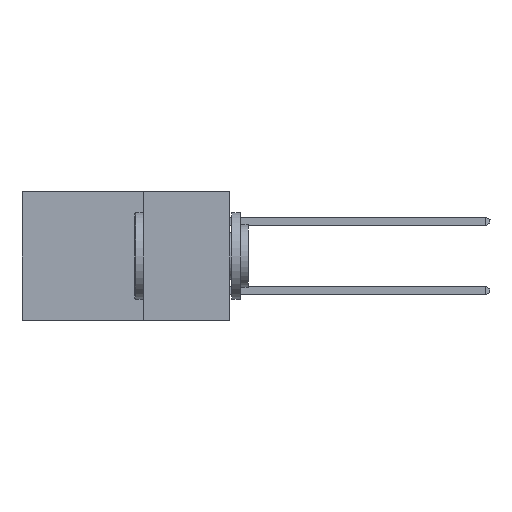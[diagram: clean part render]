
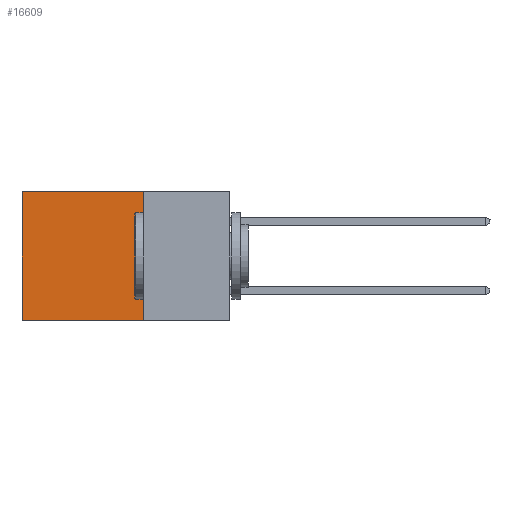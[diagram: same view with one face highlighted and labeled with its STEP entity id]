
A CAD part, left-side view. The second image highlights one B-rep face of the part: STEP entity #16609.
In plain terms, the highlighted planar face has unit normal (-1, 0, 0).
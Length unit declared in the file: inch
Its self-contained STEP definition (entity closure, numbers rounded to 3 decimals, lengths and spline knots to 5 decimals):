
#546 = DIRECTION ( 'NONE',  ( 0., 1., 0. ) ) ;
#1511 = EDGE_CURVE ( 'NONE', #17264, #19037, #10240, .T. ) ;
#3808 = CARTESIAN_POINT ( 'NONE',  ( 0.2615, 0.25, -0.37 ) ) ;
#4398 = VECTOR ( 'NONE', #15014, 39.37008 ) ;
#5291 = ORIENTED_EDGE ( 'NONE', *, *, #14490, .T. ) ;
#6304 = ORIENTED_EDGE ( 'NONE', *, *, #17550, .F. ) ;
#6436 = CARTESIAN_POINT ( 'NONE',  ( 0.2615, 0.6, -0.37 ) ) ;
#7663 = CARTESIAN_POINT ( 'NONE',  ( 0.2615, 0.25, -0.37 ) ) ;
#7667 = CARTESIAN_POINT ( 'NONE',  ( 0.2615, 0.25, 0. ) ) ;
#8010 = CARTESIAN_POINT ( 'NONE',  ( 0.2615, 0.6, 0. ) ) ;
#8348 = CARTESIAN_POINT ( 'NONE',  ( 0.2615, 0.25, 0. ) ) ;
#8584 = LINE ( 'NONE', #6436, #4398 ) ;
#10240 = LINE ( 'NONE', #3808, #11308 ) ;
#11308 = VECTOR ( 'NONE', #18964, 39.37008 ) ;
#12254 = CARTESIAN_POINT ( 'NONE',  ( 0.2615, 0.25, -0.37 ) ) ;
#12441 = VECTOR ( 'NONE', #546, 39.37008 ) ;
#12472 = LINE ( 'NONE', #27522, #13146 ) ;
#13146 = VECTOR ( 'NONE', #25366, 39.37008 ) ;
#13531 = AXIS2_PLACEMENT_3D ( 'NONE', #12254, #25421, #18827 ) ;
#14490 = EDGE_CURVE ( 'NONE', #25610, #26361, #8584, .T. ) ;
#15014 = DIRECTION ( 'NONE',  ( 0., 0., -1. ) ) ;
#15855 = CARTESIAN_POINT ( 'NONE',  ( 0.2615, 0.6, -0.37 ) ) ;
#16609 = ADVANCED_FACE ( 'NONE', ( #18974 ), #25133, .F. ) ;
#17264 = VERTEX_POINT ( 'NONE', #8348 ) ;
#17550 = EDGE_CURVE ( 'NONE', #19037, #26361, #12472, .T. ) ;
#18542 = LINE ( 'NONE', #7667, #12441 ) ;
#18827 = DIRECTION ( 'NONE',  ( 0., 0., -1. ) ) ;
#18964 = DIRECTION ( 'NONE',  ( 0., 0., -1. ) ) ;
#18974 = FACE_OUTER_BOUND ( 'NONE', #20964, .T. ) ;
#19037 = VERTEX_POINT ( 'NONE', #7663 ) ;
#20250 = EDGE_CURVE ( 'NONE', #17264, #25610, #18542, .T. ) ;
#20964 = EDGE_LOOP ( 'NONE', ( #5291, #6304, #23328, #22970 ) ) ;
#22970 = ORIENTED_EDGE ( 'NONE', *, *, #20250, .T. ) ;
#23328 = ORIENTED_EDGE ( 'NONE', *, *, #1511, .F. ) ;
#25133 = PLANE ( 'NONE',  #13531 ) ;
#25366 = DIRECTION ( 'NONE',  ( 0., 1., 0. ) ) ;
#25421 = DIRECTION ( 'NONE',  ( 1., 0., 0. ) ) ;
#25610 = VERTEX_POINT ( 'NONE', #8010 ) ;
#26361 = VERTEX_POINT ( 'NONE', #15855 ) ;
#27522 = CARTESIAN_POINT ( 'NONE',  ( 0.2615, 0.25, -0.37 ) ) ;
